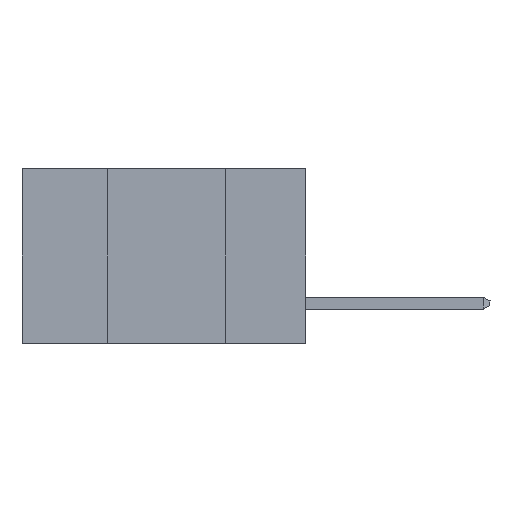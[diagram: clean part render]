
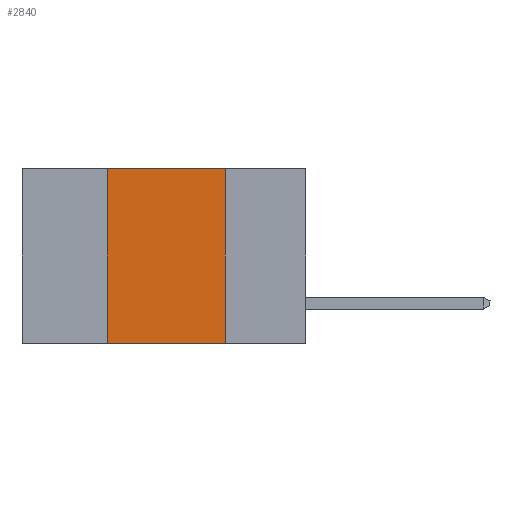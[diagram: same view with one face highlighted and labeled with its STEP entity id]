
A CAD part, left-side view. The second image highlights one B-rep face of the part: STEP entity #2840.
In plain terms, the highlighted planar face has unit normal (-1, 0, 0).
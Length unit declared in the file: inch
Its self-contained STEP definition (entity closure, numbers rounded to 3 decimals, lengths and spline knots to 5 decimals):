
#677 = CARTESIAN_POINT ( 'NONE',  ( 0., 0.42, 0. ) ) ;
#739 = EDGE_CURVE ( 'NONE', #20696, #2058, #1221, .T. ) ;
#843 = DIRECTION ( 'NONE',  ( 0., -1., 0. ) ) ;
#1221 = LINE ( 'NONE', #6308, #8720 ) ;
#2058 = VERTEX_POINT ( 'NONE', #677 ) ;
#2079 = VECTOR ( 'NONE', #843, 39.37008 ) ;
#2367 = LINE ( 'NONE', #5511, #6559 ) ;
#2840 = ADVANCED_FACE ( 'NONE', ( #25968 ), #12404, .F. ) ;
#3134 = EDGE_CURVE ( 'NONE', #20696, #6883, #7585, .T. ) ;
#3136 = CARTESIAN_POINT ( 'NONE',  ( 0., 0.6, 0. ) ) ;
#5511 = CARTESIAN_POINT ( 'NONE',  ( 0., 0.17, 0. ) ) ;
#6308 = CARTESIAN_POINT ( 'NONE',  ( 0., 0.42, 0. ) ) ;
#6559 = VECTOR ( 'NONE', #26445, 39.37008 ) ;
#6883 = VERTEX_POINT ( 'NONE', #7919 ) ;
#7324 = VECTOR ( 'NONE', #23824, 39.37008 ) ;
#7517 = EDGE_LOOP ( 'NONE', ( #13365, #21724, #21453, #9074 ) ) ;
#7585 = LINE ( 'NONE', #13319, #2079 ) ;
#7919 = CARTESIAN_POINT ( 'NONE',  ( 0., 0.17, -0.37 ) ) ;
#8720 = VECTOR ( 'NONE', #12599, 39.37008 ) ;
#9074 = ORIENTED_EDGE ( 'NONE', *, *, #3134, .T. ) ;
#11672 = VERTEX_POINT ( 'NONE', #14323 ) ;
#12404 = PLANE ( 'NONE',  #18456 ) ;
#12599 = DIRECTION ( 'NONE',  ( 0., 0., 1. ) ) ;
#13319 = CARTESIAN_POINT ( 'NONE',  ( 0., 0.6, -0.37 ) ) ;
#13365 = ORIENTED_EDGE ( 'NONE', *, *, #24741, .F. ) ;
#14323 = CARTESIAN_POINT ( 'NONE',  ( 0., 0.17, 0. ) ) ;
#14526 = DIRECTION ( 'NONE',  ( 1., 0., 0. ) ) ;
#15637 = EDGE_CURVE ( 'NONE', #2058, #11672, #21728, .T. ) ;
#18456 = AXIS2_PLACEMENT_3D ( 'NONE', #25317, #14526, #25229 ) ;
#20696 = VERTEX_POINT ( 'NONE', #21854 ) ;
#21453 = ORIENTED_EDGE ( 'NONE', *, *, #739, .F. ) ;
#21724 = ORIENTED_EDGE ( 'NONE', *, *, #15637, .F. ) ;
#21728 = LINE ( 'NONE', #3136, #7324 ) ;
#21854 = CARTESIAN_POINT ( 'NONE',  ( 0., 0.42, -0.37 ) ) ;
#23824 = DIRECTION ( 'NONE',  ( 0., -1., 0. ) ) ;
#24741 = EDGE_CURVE ( 'NONE', #11672, #6883, #2367, .T. ) ;
#25229 = DIRECTION ( 'NONE',  ( 0., 0., -1. ) ) ;
#25317 = CARTESIAN_POINT ( 'NONE',  ( 0., 0.6, 0. ) ) ;
#25968 = FACE_OUTER_BOUND ( 'NONE', #7517, .T. ) ;
#26445 = DIRECTION ( 'NONE',  ( 0., 0., -1. ) ) ;
